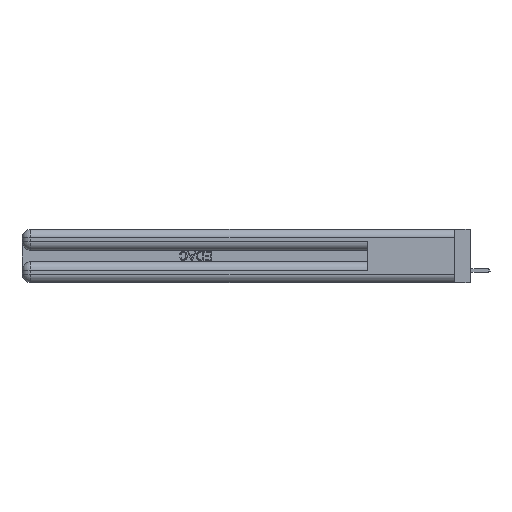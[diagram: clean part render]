
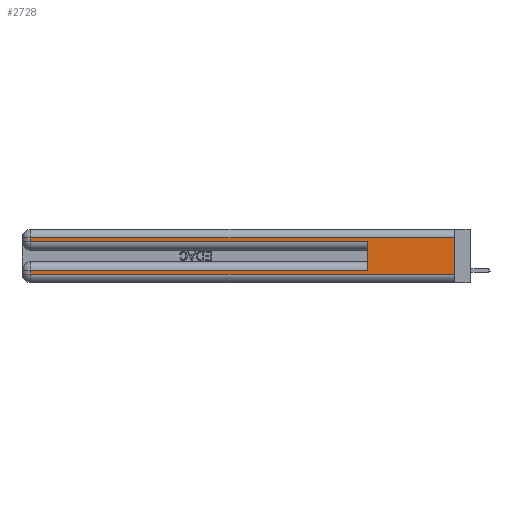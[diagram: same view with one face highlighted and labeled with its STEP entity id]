
A CAD part, left-side view. The second image highlights one B-rep face of the part: STEP entity #2728.
In plain terms, the highlighted planar face has unit normal (-1, 0, 0).
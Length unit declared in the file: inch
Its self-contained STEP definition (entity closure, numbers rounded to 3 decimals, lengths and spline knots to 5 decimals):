
#524 = ORIENTED_EDGE ( 'NONE', *, *, #37349, .T. ) ;
#1323 = LINE ( 'NONE', #37828, #5678 ) ;
#2678 = LINE ( 'NONE', #28505, #6990 ) ;
#2728 = ADVANCED_FACE ( 'NONE', ( #39983 ), #43569, .F. ) ;
#2878 = CARTESIAN_POINT ( 'NONE',  ( 0., 2.94, 0.37 ) ) ;
#3965 = VECTOR ( 'NONE', #16649, 39.37008 ) ;
#4178 = ORIENTED_EDGE ( 'NONE', *, *, #16167, .T. ) ;
#4577 = VERTEX_POINT ( 'NONE', #23377 ) ;
#4885 = DIRECTION ( 'NONE',  ( 0., 0., -1. ) ) ;
#5678 = VECTOR ( 'NONE', #20765, 39.37008 ) ;
#6708 = LINE ( 'NONE', #2878, #3965 ) ;
#6737 = ORIENTED_EDGE ( 'NONE', *, *, #34214, .T. ) ;
#6990 = VECTOR ( 'NONE', #35401, 39.37008 ) ;
#7976 = VECTOR ( 'NONE', #22909, 39.37008 ) ;
#8230 = VECTOR ( 'NONE', #4885, 39.37008 ) ;
#8324 = CARTESIAN_POINT ( 'NONE',  ( 0., 0., 0.37 ) ) ;
#9192 = CARTESIAN_POINT ( 'NONE',  ( 0., 0., 0.37 ) ) ;
#9572 = AXIS2_PLACEMENT_3D ( 'NONE', #9192, #36852, #13117 ) ;
#9732 = VERTEX_POINT ( 'NONE', #18013 ) ;
#11411 = LINE ( 'NONE', #26023, #16232 ) ;
#13110 = LINE ( 'NONE', #8324, #8230 ) ;
#13117 = DIRECTION ( 'NONE',  ( 0., 0., -1. ) ) ;
#14156 = VERTEX_POINT ( 'NONE', #14580 ) ;
#14361 = EDGE_CURVE ( 'NONE', #36138, #22701, #2678, .T. ) ;
#14432 = CARTESIAN_POINT ( 'NONE',  ( 0., 0., 0.06 ) ) ;
#14580 = CARTESIAN_POINT ( 'NONE',  ( 0., 0., 0.06 ) ) ;
#14841 = CARTESIAN_POINT ( 'NONE',  ( 0., 0.6, 0.085 ) ) ;
#15150 = VERTEX_POINT ( 'NONE', #14841 ) ;
#15893 = DIRECTION ( 'NONE',  ( 0., 0., 1. ) ) ;
#16167 = EDGE_CURVE ( 'NONE', #4577, #9732, #37769, .T. ) ;
#16232 = VECTOR ( 'NONE', #15893, 39.37008 ) ;
#16649 = DIRECTION ( 'NONE',  ( 0., 0., -1. ) ) ;
#17596 = LINE ( 'NONE', #40131, #7976 ) ;
#17924 = ORIENTED_EDGE ( 'NONE', *, *, #14361, .T. ) ;
#18013 = CARTESIAN_POINT ( 'NONE',  ( 0., 0.6, 0.285 ) ) ;
#18417 = VECTOR ( 'NONE', #21694, 39.37008 ) ;
#18631 = EDGE_CURVE ( 'NONE', #15150, #9732, #11411, .T. ) ;
#20765 = DIRECTION ( 'NONE',  ( 0., 0., -1. ) ) ;
#21694 = DIRECTION ( 'NONE',  ( 0., -1., 0. ) ) ;
#22701 = VERTEX_POINT ( 'NONE', #41438 ) ;
#22909 = DIRECTION ( 'NONE',  ( 0., 1., 0. ) ) ;
#23377 = CARTESIAN_POINT ( 'NONE',  ( 0., 2.94, 0.285 ) ) ;
#25227 = VERTEX_POINT ( 'NONE', #34905 ) ;
#26023 = CARTESIAN_POINT ( 'NONE',  ( 0., 0.6, 0.145 ) ) ;
#27303 = ORIENTED_EDGE ( 'NONE', *, *, #41628, .F. ) ;
#27318 = CARTESIAN_POINT ( 'NONE',  ( 0., 0., 0.31 ) ) ;
#27529 = LINE ( 'NONE', #14432, #18417 ) ;
#28505 = CARTESIAN_POINT ( 'NONE',  ( 0., 0., 0.31 ) ) ;
#28967 = EDGE_CURVE ( 'NONE', #25227, #14156, #27529, .T. ) ;
#30360 = ORIENTED_EDGE ( 'NONE', *, *, #18631, .F. ) ;
#30862 = ORIENTED_EDGE ( 'NONE', *, *, #28967, .T. ) ;
#34214 = EDGE_CURVE ( 'NONE', #15150, #38107, #17596, .T. ) ;
#34905 = CARTESIAN_POINT ( 'NONE',  ( 0., 2.94, 0.06 ) ) ;
#35110 = VECTOR ( 'NONE', #42655, 39.37008 ) ;
#35401 = DIRECTION ( 'NONE',  ( 0., 1., 0. ) ) ;
#36138 = VERTEX_POINT ( 'NONE', #27318 ) ;
#36852 = DIRECTION ( 'NONE',  ( 1., 0., 0. ) ) ;
#36869 = ORIENTED_EDGE ( 'NONE', *, *, #40865, .T. ) ;
#37349 = EDGE_CURVE ( 'NONE', #38107, #25227, #6708, .T. ) ;
#37769 = LINE ( 'NONE', #42060, #35110 ) ;
#37828 = CARTESIAN_POINT ( 'NONE',  ( 0., 2.94, 0.37 ) ) ;
#38107 = VERTEX_POINT ( 'NONE', #40372 ) ;
#39983 = FACE_OUTER_BOUND ( 'NONE', #42727, .T. ) ;
#40131 = CARTESIAN_POINT ( 'NONE',  ( 0., 0., 0.085 ) ) ;
#40372 = CARTESIAN_POINT ( 'NONE',  ( 0., 2.94, 0.085 ) ) ;
#40865 = EDGE_CURVE ( 'NONE', #22701, #4577, #1323, .T. ) ;
#41438 = CARTESIAN_POINT ( 'NONE',  ( 0., 2.94, 0.31 ) ) ;
#41628 = EDGE_CURVE ( 'NONE', #36138, #14156, #13110, .T. ) ;
#42060 = CARTESIAN_POINT ( 'NONE',  ( 0., 0., 0.285 ) ) ;
#42655 = DIRECTION ( 'NONE',  ( 0., -1., 0. ) ) ;
#42727 = EDGE_LOOP ( 'NONE', ( #27303, #17924, #36869, #4178, #30360, #6737, #524, #30862 ) ) ;
#43569 = PLANE ( 'NONE',  #9572 ) ;
